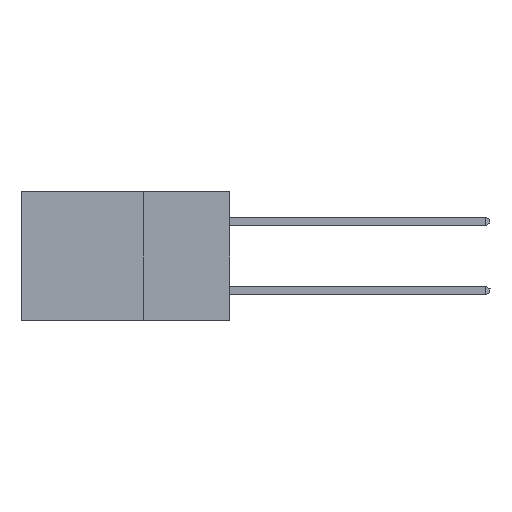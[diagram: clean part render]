
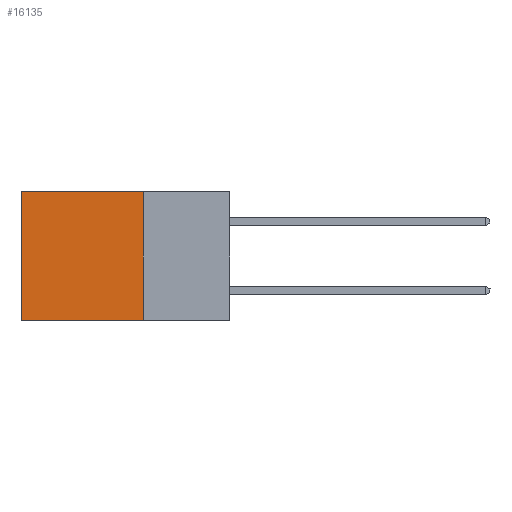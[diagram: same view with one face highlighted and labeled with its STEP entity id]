
A CAD part, left-side view. The second image highlights one B-rep face of the part: STEP entity #16135.
In plain terms, the highlighted planar face has unit normal (-1, 0, 0).
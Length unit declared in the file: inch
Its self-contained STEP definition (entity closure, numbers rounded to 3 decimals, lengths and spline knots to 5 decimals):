
#394 = LINE ( 'NONE', #11338, #15573 ) ;
#1381 = ORIENTED_EDGE ( 'NONE', *, *, #18220, .T. ) ;
#1583 = EDGE_CURVE ( 'NONE', #22845, #14692, #19208, .T. ) ;
#1722 = DIRECTION ( 'NONE',  ( 0., 0., -1. ) ) ;
#3533 = CARTESIAN_POINT ( 'NONE',  ( 0.2615, 0.6, -0.37 ) ) ;
#4254 = CARTESIAN_POINT ( 'NONE',  ( 0.2615, 0.25, -0.37 ) ) ;
#4389 = CARTESIAN_POINT ( 'NONE',  ( 0.2615, 0.25, 0. ) ) ;
#4435 = AXIS2_PLACEMENT_3D ( 'NONE', #20545, #9759, #22318 ) ;
#5711 = CARTESIAN_POINT ( 'NONE',  ( 0.2615, 0.25, 0. ) ) ;
#6191 = CARTESIAN_POINT ( 'NONE',  ( 0.2615, 0.6, -0.37 ) ) ;
#8552 = LINE ( 'NONE', #4254, #13347 ) ;
#9759 = DIRECTION ( 'NONE',  ( 1., 0., 0. ) ) ;
#9986 = ORIENTED_EDGE ( 'NONE', *, *, #16483, .F. ) ;
#11338 = CARTESIAN_POINT ( 'NONE',  ( 0.2615, 0.25, -0.37 ) ) ;
#11781 = ORIENTED_EDGE ( 'NONE', *, *, #22755, .F. ) ;
#13016 = VECTOR ( 'NONE', #1722, 39.37008 ) ;
#13347 = VECTOR ( 'NONE', #16919, 39.37008 ) ;
#14300 = DIRECTION ( 'NONE',  ( 0., 1., 0. ) ) ;
#14692 = VERTEX_POINT ( 'NONE', #18355 ) ;
#15118 = EDGE_LOOP ( 'NONE', ( #1381, #11781, #9986, #18103 ) ) ;
#15168 = PLANE ( 'NONE',  #4435 ) ;
#15573 = VECTOR ( 'NONE', #18618, 39.37008 ) ;
#15945 = FACE_OUTER_BOUND ( 'NONE', #15118, .T. ) ;
#16135 = ADVANCED_FACE ( 'NONE', ( #15945 ), #15168, .F. ) ;
#16371 = VERTEX_POINT ( 'NONE', #16610 ) ;
#16483 = EDGE_CURVE ( 'NONE', #22845, #16371, #8552, .T. ) ;
#16610 = CARTESIAN_POINT ( 'NONE',  ( 0.2615, 0.25, -0.37 ) ) ;
#16919 = DIRECTION ( 'NONE',  ( 0., 0., -1. ) ) ;
#18103 = ORIENTED_EDGE ( 'NONE', *, *, #1583, .T. ) ;
#18220 = EDGE_CURVE ( 'NONE', #14692, #21318, #22540, .T. ) ;
#18355 = CARTESIAN_POINT ( 'NONE',  ( 0.2615, 0.6, 0. ) ) ;
#18618 = DIRECTION ( 'NONE',  ( 0., 1., 0. ) ) ;
#18661 = VECTOR ( 'NONE', #14300, 39.37008 ) ;
#19208 = LINE ( 'NONE', #5711, #18661 ) ;
#20545 = CARTESIAN_POINT ( 'NONE',  ( 0.2615, 0.25, -0.37 ) ) ;
#21318 = VERTEX_POINT ( 'NONE', #6191 ) ;
#22318 = DIRECTION ( 'NONE',  ( 0., 0., -1. ) ) ;
#22540 = LINE ( 'NONE', #3533, #13016 ) ;
#22755 = EDGE_CURVE ( 'NONE', #16371, #21318, #394, .T. ) ;
#22845 = VERTEX_POINT ( 'NONE', #4389 ) ;
